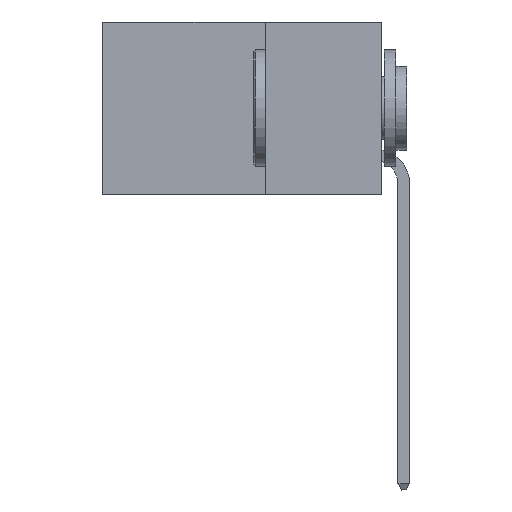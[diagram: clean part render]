
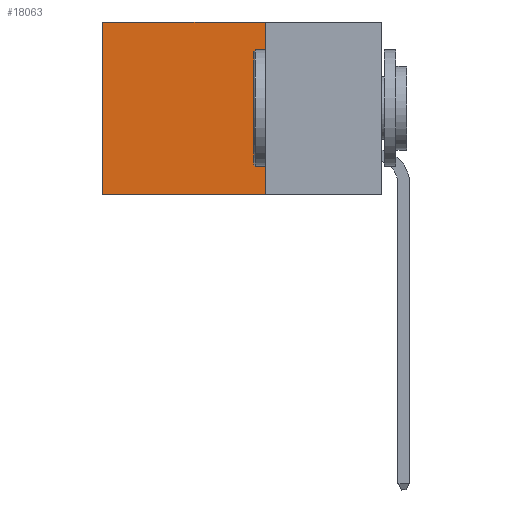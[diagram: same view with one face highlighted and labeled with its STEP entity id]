
A CAD part, left-side view. The second image highlights one B-rep face of the part: STEP entity #18063.
In plain terms, the highlighted planar face has unit normal (-1, 0, 0).
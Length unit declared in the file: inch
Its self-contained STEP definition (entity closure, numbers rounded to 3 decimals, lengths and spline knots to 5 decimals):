
#239 = VECTOR ( 'NONE', #17984, 39.37008 ) ;
#650 = CARTESIAN_POINT ( 'NONE',  ( 0.2875, 0.25, 0. ) ) ;
#1265 = FACE_OUTER_BOUND ( 'NONE', #17967, .T. ) ;
#2001 = DIRECTION ( 'NONE',  ( 1., 0., 0. ) ) ;
#2560 = EDGE_CURVE ( 'NONE', #6950, #8266, #10351, .T. ) ;
#2842 = LINE ( 'NONE', #17739, #17938 ) ;
#3683 = AXIS2_PLACEMENT_3D ( 'NONE', #650, #2001, #14500 ) ;
#4392 = VERTEX_POINT ( 'NONE', #10672 ) ;
#5443 = DIRECTION ( 'NONE',  ( 0., 1., 0. ) ) ;
#6422 = LINE ( 'NONE', #16582, #239 ) ;
#6950 = VERTEX_POINT ( 'NONE', #15573 ) ;
#7401 = CARTESIAN_POINT ( 'NONE',  ( 0.2875, 0.25, 0. ) ) ;
#7423 = CARTESIAN_POINT ( 'NONE',  ( 0.2875, 0.6, 0. ) ) ;
#7691 = LINE ( 'NONE', #7423, #16148 ) ;
#8266 = VERTEX_POINT ( 'NONE', #8364 ) ;
#8364 = CARTESIAN_POINT ( 'NONE',  ( 0.2875, 0.6, -0.37 ) ) ;
#8569 = EDGE_CURVE ( 'NONE', #4392, #8266, #7691, .T. ) ;
#8728 = EDGE_CURVE ( 'NONE', #17948, #6950, #2842, .T. ) ;
#9001 = PLANE ( 'NONE',  #3683 ) ;
#10351 = LINE ( 'NONE', #17877, #16428 ) ;
#10530 = DIRECTION ( 'NONE',  ( 0., 0., -1. ) ) ;
#10672 = CARTESIAN_POINT ( 'NONE',  ( 0.2875, 0.6, 0. ) ) ;
#10929 = ORIENTED_EDGE ( 'NONE', *, *, #8728, .F. ) ;
#14500 = DIRECTION ( 'NONE',  ( 0., 0., -1. ) ) ;
#14740 = ORIENTED_EDGE ( 'NONE', *, *, #2560, .F. ) ;
#15365 = ORIENTED_EDGE ( 'NONE', *, *, #16669, .T. ) ;
#15573 = CARTESIAN_POINT ( 'NONE',  ( 0.2875, 0.25, -0.37 ) ) ;
#16148 = VECTOR ( 'NONE', #10530, 39.37008 ) ;
#16428 = VECTOR ( 'NONE', #5443, 39.37008 ) ;
#16499 = DIRECTION ( 'NONE',  ( 0., 0., -1. ) ) ;
#16582 = CARTESIAN_POINT ( 'NONE',  ( 0.2875, 0.25, 0. ) ) ;
#16669 = EDGE_CURVE ( 'NONE', #17948, #4392, #6422, .T. ) ;
#17636 = ORIENTED_EDGE ( 'NONE', *, *, #8569, .T. ) ;
#17739 = CARTESIAN_POINT ( 'NONE',  ( 0.2875, 0.25, 0. ) ) ;
#17877 = CARTESIAN_POINT ( 'NONE',  ( 0.2875, 0.25, -0.37 ) ) ;
#17938 = VECTOR ( 'NONE', #16499, 39.37008 ) ;
#17948 = VERTEX_POINT ( 'NONE', #7401 ) ;
#17967 = EDGE_LOOP ( 'NONE', ( #17636, #14740, #10929, #15365 ) ) ;
#17984 = DIRECTION ( 'NONE',  ( 0., 1., 0. ) ) ;
#18063 = ADVANCED_FACE ( 'NONE', ( #1265 ), #9001, .F. ) ;
